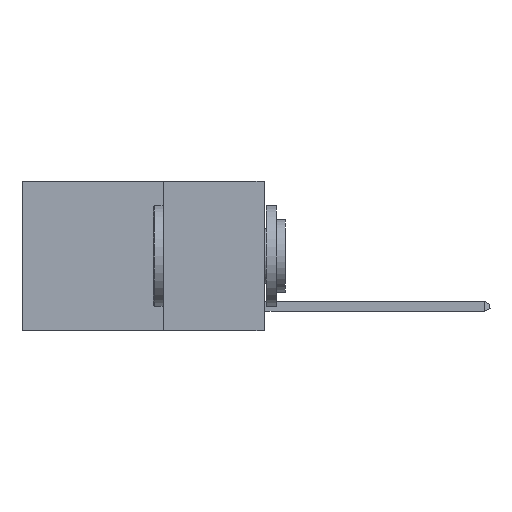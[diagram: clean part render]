
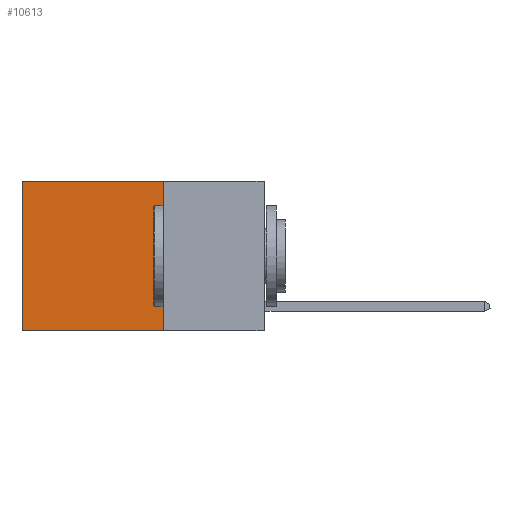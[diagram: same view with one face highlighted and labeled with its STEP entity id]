
A CAD part, left-side view. The second image highlights one B-rep face of the part: STEP entity #10613.
In plain terms, the highlighted planar face has unit normal (-1, 0, 0).
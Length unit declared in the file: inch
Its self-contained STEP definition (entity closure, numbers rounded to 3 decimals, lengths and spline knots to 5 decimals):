
#23 = LINE ( 'NONE', #4868, #10030 ) ;
#809 = EDGE_LOOP ( 'NONE', ( #3352, #10973, #6688, #15055 ) ) ;
#1118 = VECTOR ( 'NONE', #12709, 39.37008 ) ;
#1214 = CARTESIAN_POINT ( 'NONE',  ( 0.2625, 0.25, -0.37 ) ) ;
#1347 = VERTEX_POINT ( 'NONE', #1214 ) ;
#1394 = VECTOR ( 'NONE', #14121, 39.37008 ) ;
#2060 = EDGE_CURVE ( 'NONE', #2417, #7473, #14157, .T. ) ;
#2104 = DIRECTION ( 'NONE',  ( 0., 0., -1. ) ) ;
#2229 = CARTESIAN_POINT ( 'NONE',  ( 0.2625, 0.25, 0. ) ) ;
#2417 = VERTEX_POINT ( 'NONE', #2229 ) ;
#3352 = ORIENTED_EDGE ( 'NONE', *, *, #6786, .T. ) ;
#4502 = EDGE_CURVE ( 'NONE', #1347, #11406, #6009, .T. ) ;
#4868 = CARTESIAN_POINT ( 'NONE',  ( 0.2625, 0.25, 0. ) ) ;
#5410 = CARTESIAN_POINT ( 'NONE',  ( 0.2625, 0.6, -0.37 ) ) ;
#5903 = VECTOR ( 'NONE', #11650, 39.37008 ) ;
#6009 = LINE ( 'NONE', #13768, #1118 ) ;
#6688 = ORIENTED_EDGE ( 'NONE', *, *, #14110, .F. ) ;
#6786 = EDGE_CURVE ( 'NONE', #7473, #11406, #14911, .T. ) ;
#7473 = VERTEX_POINT ( 'NONE', #11254 ) ;
#10030 = VECTOR ( 'NONE', #14434, 39.37008 ) ;
#10401 = CARTESIAN_POINT ( 'NONE',  ( 0.2625, 0.25, 0. ) ) ;
#10534 = CARTESIAN_POINT ( 'NONE',  ( 0.2625, 0.6, 0. ) ) ;
#10613 = ADVANCED_FACE ( 'NONE', ( #12922 ), #14033, .F. ) ;
#10691 = AXIS2_PLACEMENT_3D ( 'NONE', #11898, #13110, #2104 ) ;
#10973 = ORIENTED_EDGE ( 'NONE', *, *, #4502, .F. ) ;
#11254 = CARTESIAN_POINT ( 'NONE',  ( 0.2625, 0.6, 0. ) ) ;
#11406 = VERTEX_POINT ( 'NONE', #5410 ) ;
#11650 = DIRECTION ( 'NONE',  ( 0., 1., 0. ) ) ;
#11898 = CARTESIAN_POINT ( 'NONE',  ( 0.2625, 0.25, 0. ) ) ;
#12709 = DIRECTION ( 'NONE',  ( 0., 1., 0. ) ) ;
#12922 = FACE_OUTER_BOUND ( 'NONE', #809, .T. ) ;
#13110 = DIRECTION ( 'NONE',  ( 1., 0., 0. ) ) ;
#13768 = CARTESIAN_POINT ( 'NONE',  ( 0.2625, 0.25, -0.37 ) ) ;
#14033 = PLANE ( 'NONE',  #10691 ) ;
#14110 = EDGE_CURVE ( 'NONE', #2417, #1347, #23, .T. ) ;
#14121 = DIRECTION ( 'NONE',  ( 0., 0., -1. ) ) ;
#14157 = LINE ( 'NONE', #10401, #5903 ) ;
#14434 = DIRECTION ( 'NONE',  ( 0., 0., -1. ) ) ;
#14911 = LINE ( 'NONE', #10534, #1394 ) ;
#15055 = ORIENTED_EDGE ( 'NONE', *, *, #2060, .T. ) ;
